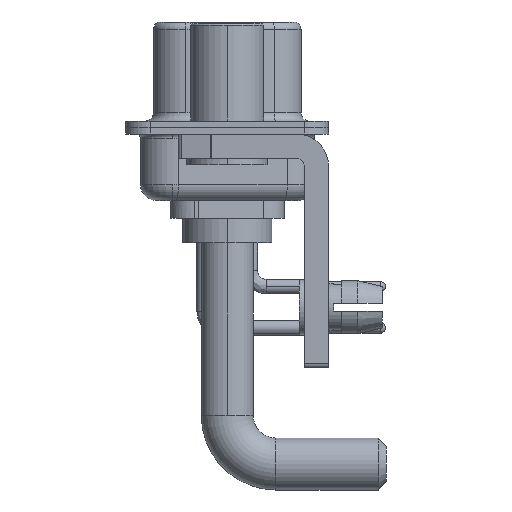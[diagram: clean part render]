
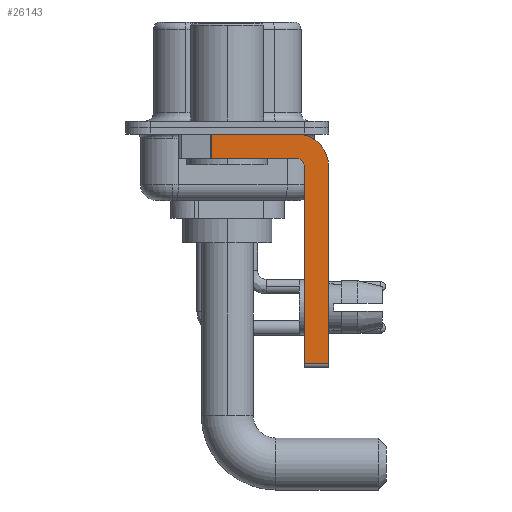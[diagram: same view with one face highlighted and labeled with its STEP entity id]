
A CAD part, left-side view. The second image highlights one B-rep face of the part: STEP entity #26143.
In plain terms, the highlighted planar face has unit normal (-1, 0, 0).
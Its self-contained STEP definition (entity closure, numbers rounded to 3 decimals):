
#462 = DIRECTION ( 'NONE',  ( 1., 0., 0. ) ) ;
#533 = ORIENTED_EDGE ( 'NONE', *, *, #19900, .F. ) ;
#897 = ORIENTED_EDGE ( 'NONE', *, *, #7695, .F. ) ;
#958 = LINE ( 'NONE', #13431, #13535 ) ;
#1001 = FACE_OUTER_BOUND ( 'NONE', #8691, .T. ) ;
#1780 = CARTESIAN_POINT ( 'NONE',  ( -2.9, -4.75, -2.4 ) ) ;
#2140 = AXIS2_PLACEMENT_3D ( 'NONE', #19145, #23508, #25487 ) ;
#2915 = CARTESIAN_POINT ( 'NONE',  ( -2.9, -4.75, -14.55 ) ) ;
#3184 = DIRECTION ( 'NONE',  ( 0., 0., 1. ) ) ;
#3728 = CARTESIAN_POINT ( 'NONE',  ( -2.9, -4.25, -14.55 ) ) ;
#7242 = CARTESIAN_POINT ( 'NONE',  ( -2.9, -4.25, -2.4 ) ) ;
#7695 = EDGE_CURVE ( 'NONE', #23215, #13249, #19388, .T. ) ;
#8224 = DIRECTION ( 'NONE',  ( 0., 1., 0. ) ) ;
#8691 = EDGE_LOOP ( 'NONE', ( #17346, #20290, #533, #16820, #897, #13583, #24879, #16811 ) ) ;
#8978 = DIRECTION ( 'NONE',  ( 0., 0., -1. ) ) ;
#9010 = VERTEX_POINT ( 'NONE', #23346 ) ;
#9021 = DIRECTION ( 'NONE',  ( 0., 0., 1. ) ) ;
#9140 = DIRECTION ( 'NONE',  ( 0., 0., -1. ) ) ;
#9296 = VERTEX_POINT ( 'NONE', #11405 ) ;
#9683 = EDGE_CURVE ( 'NONE', #22762, #9296, #16147, .T. ) ;
#10026 = LINE ( 'NONE', #3728, #10746 ) ;
#10746 = VECTOR ( 'NONE', #25049, 1000. ) ;
#11405 = CARTESIAN_POINT ( 'NONE',  ( -2.9, -6.25, -14.55 ) ) ;
#11625 = CARTESIAN_POINT ( 'NONE',  ( -2.9, -6.25, -2.4 ) ) ;
#11859 = DIRECTION ( 'NONE',  ( 0., -1., 0. ) ) ;
#13088 = CARTESIAN_POINT ( 'NONE',  ( -2.9, -4.75, -14.8 ) ) ;
#13249 = VERTEX_POINT ( 'NONE', #1780 ) ;
#13431 = CARTESIAN_POINT ( 'NONE',  ( -2.9, 3., -0.4 ) ) ;
#13479 = VECTOR ( 'NONE', #8224, 1000. ) ;
#13535 = VECTOR ( 'NONE', #11859, 1000. ) ;
#13583 = ORIENTED_EDGE ( 'NONE', *, *, #19404, .T. ) ;
#14217 = CIRCLE ( 'NONE', #2140, 2. ) ;
#14791 = VERTEX_POINT ( 'NONE', #20700 ) ;
#14882 = VECTOR ( 'NONE', #8978, 1000. ) ;
#14913 = EDGE_CURVE ( 'NONE', #14791, #22762, #14217, .T. ) ;
#15154 = LINE ( 'NONE', #23707, #14882 ) ;
#16047 = VERTEX_POINT ( 'NONE', #26397 ) ;
#16147 = LINE ( 'NONE', #22027, #24807 ) ;
#16811 = ORIENTED_EDGE ( 'NONE', *, *, #14913, .F. ) ;
#16820 = ORIENTED_EDGE ( 'NONE', *, *, #21894, .F. ) ;
#17152 = CIRCLE ( 'NONE', #26109, 0.5 ) ;
#17284 = AXIS2_PLACEMENT_3D ( 'NONE', #26664, #462, #22851 ) ;
#17346 = ORIENTED_EDGE ( 'NONE', *, *, #23186, .F. ) ;
#18093 = PLANE ( 'NONE',  #17284 ) ;
#18868 = LINE ( 'NONE', #27454, #13479 ) ;
#19145 = CARTESIAN_POINT ( 'NONE',  ( -2.9, -4.25, -2.4 ) ) ;
#19388 = LINE ( 'NONE', #13088, #24729 ) ;
#19404 = EDGE_CURVE ( 'NONE', #23215, #9296, #10026, .T. ) ;
#19900 = EDGE_CURVE ( 'NONE', #9010, #23011, #18868, .T. ) ;
#20274 = DIRECTION ( 'NONE',  ( -1., 0., 0. ) ) ;
#20290 = ORIENTED_EDGE ( 'NONE', *, *, #21285, .T. ) ;
#20700 = CARTESIAN_POINT ( 'NONE',  ( -2.9, -4.25, -0.4 ) ) ;
#21285 = EDGE_CURVE ( 'NONE', #16047, #23011, #15154, .T. ) ;
#21894 = EDGE_CURVE ( 'NONE', #13249, #9010, #17152, .T. ) ;
#22027 = CARTESIAN_POINT ( 'NONE',  ( -2.9, -6.25, -2.4 ) ) ;
#22762 = VERTEX_POINT ( 'NONE', #11625 ) ;
#22851 = DIRECTION ( 'NONE',  ( 0., 0., -1. ) ) ;
#23011 = VERTEX_POINT ( 'NONE', #25651 ) ;
#23186 = EDGE_CURVE ( 'NONE', #16047, #14791, #958, .T. ) ;
#23215 = VERTEX_POINT ( 'NONE', #2915 ) ;
#23346 = CARTESIAN_POINT ( 'NONE',  ( -2.9, -4.25, -1.9 ) ) ;
#23508 = DIRECTION ( 'NONE',  ( 1., 0., 0. ) ) ;
#23707 = CARTESIAN_POINT ( 'NONE',  ( -2.9, 0.978, -1.9 ) ) ;
#24729 = VECTOR ( 'NONE', #9021, 1000. ) ;
#24807 = VECTOR ( 'NONE', #9140, 1000. ) ;
#24879 = ORIENTED_EDGE ( 'NONE', *, *, #9683, .F. ) ;
#25049 = DIRECTION ( 'NONE',  ( 0., -1., 0. ) ) ;
#25487 = DIRECTION ( 'NONE',  ( 0., 0., -1. ) ) ;
#25651 = CARTESIAN_POINT ( 'NONE',  ( -2.9, 0.978, -1.9 ) ) ;
#26109 = AXIS2_PLACEMENT_3D ( 'NONE', #7242, #20274, #3184 ) ;
#26143 = ADVANCED_FACE ( 'NONE', ( #1001 ), #18093, .F. ) ;
#26397 = CARTESIAN_POINT ( 'NONE',  ( -2.9, 0.978, -0.4 ) ) ;
#26664 = CARTESIAN_POINT ( 'NONE',  ( -2.9, -4.25, -2.4 ) ) ;
#27454 = CARTESIAN_POINT ( 'NONE',  ( -2.9, -4.25, -1.9 ) ) ;
